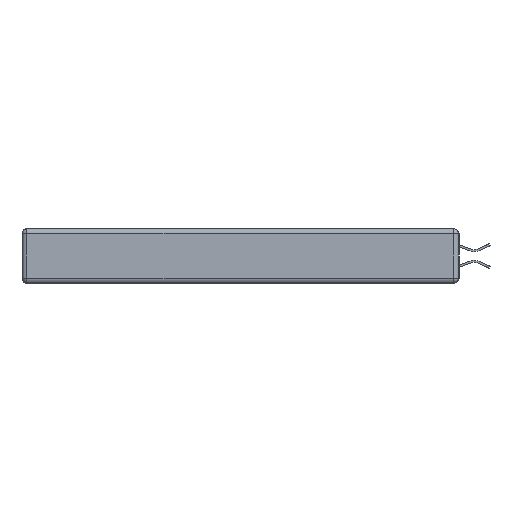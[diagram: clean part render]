
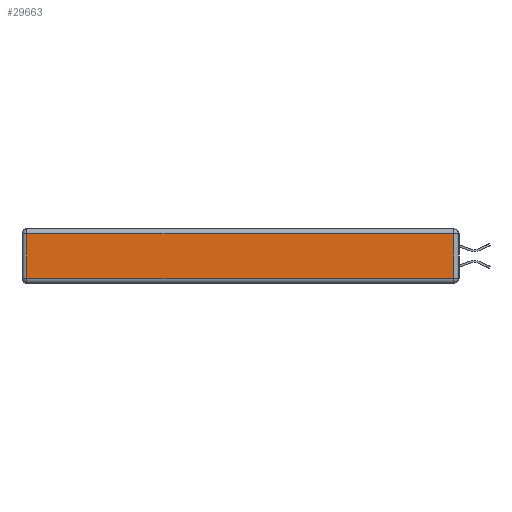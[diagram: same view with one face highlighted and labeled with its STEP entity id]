
A CAD part, left-side view. The second image highlights one B-rep face of the part: STEP entity #29663.
In plain terms, the highlighted planar face has unit normal (-1, 0, 0).
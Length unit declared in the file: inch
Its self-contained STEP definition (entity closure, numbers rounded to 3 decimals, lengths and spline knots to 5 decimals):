
#372 = PLANE ( 'NONE',  #14705 ) ;
#2803 = VECTOR ( 'NONE', #15048, 39.37008 ) ;
#2968 = EDGE_CURVE ( 'NONE', #24966, #3845, #12793, .T. ) ;
#3476 = VERTEX_POINT ( 'NONE', #5965 ) ;
#3845 = VERTEX_POINT ( 'NONE', #25146 ) ;
#5075 = CARTESIAN_POINT ( 'NONE',  ( 0., 2.72, -0.03 ) ) ;
#5227 = VECTOR ( 'NONE', #9031, 39.37008 ) ;
#5965 = CARTESIAN_POINT ( 'NONE',  ( 0., 0.03, -0.03 ) ) ;
#9031 = DIRECTION ( 'NONE',  ( 0., 1., 0. ) ) ;
#9465 = ORIENTED_EDGE ( 'NONE', *, *, #25008, .T. ) ;
#9790 = LINE ( 'NONE', #11394, #18940 ) ;
#9912 = EDGE_CURVE ( 'NONE', #3845, #15515, #18868, .T. ) ;
#10334 = EDGE_LOOP ( 'NONE', ( #23187, #9465, #24791, #19165 ) ) ;
#10374 = CARTESIAN_POINT ( 'NONE',  ( 0., 0., -0.313 ) ) ;
#10890 = FACE_OUTER_BOUND ( 'NONE', #10334, .T. ) ;
#11394 = CARTESIAN_POINT ( 'NONE',  ( 0., 0.03, -0.343 ) ) ;
#11573 = CARTESIAN_POINT ( 'NONE',  ( 0., 0.03, -0.313 ) ) ;
#11800 = DIRECTION ( 'NONE',  ( 0., 0., 1. ) ) ;
#12793 = LINE ( 'NONE', #19928, #14259 ) ;
#12969 = DIRECTION ( 'NONE',  ( 0., 0., -1. ) ) ;
#14259 = VECTOR ( 'NONE', #12969, 39.37008 ) ;
#14705 = AXIS2_PLACEMENT_3D ( 'NONE', #17268, #19738, #26059 ) ;
#15048 = DIRECTION ( 'NONE',  ( 0., -1., 0. ) ) ;
#15515 = VERTEX_POINT ( 'NONE', #11573 ) ;
#17268 = CARTESIAN_POINT ( 'NONE',  ( 0., 0., -0.343 ) ) ;
#17590 = LINE ( 'NONE', #20454, #5227 ) ;
#18868 = LINE ( 'NONE', #10374, #2803 ) ;
#18940 = VECTOR ( 'NONE', #11800, 39.37008 ) ;
#19165 = ORIENTED_EDGE ( 'NONE', *, *, #2968, .T. ) ;
#19738 = DIRECTION ( 'NONE',  ( -1., 0., 0. ) ) ;
#19928 = CARTESIAN_POINT ( 'NONE',  ( 0., 2.72, -0.343 ) ) ;
#20454 = CARTESIAN_POINT ( 'NONE',  ( 0., 2.75, -0.03 ) ) ;
#23187 = ORIENTED_EDGE ( 'NONE', *, *, #9912, .T. ) ;
#23268 = EDGE_CURVE ( 'NONE', #3476, #24966, #17590, .T. ) ;
#24791 = ORIENTED_EDGE ( 'NONE', *, *, #23268, .T. ) ;
#24966 = VERTEX_POINT ( 'NONE', #5075 ) ;
#25008 = EDGE_CURVE ( 'NONE', #15515, #3476, #9790, .T. ) ;
#25146 = CARTESIAN_POINT ( 'NONE',  ( 0., 2.72, -0.313 ) ) ;
#26059 = DIRECTION ( 'NONE',  ( 0., 0., 1. ) ) ;
#29663 = ADVANCED_FACE ( 'NONE', ( #10890 ), #372, .T. ) ;
